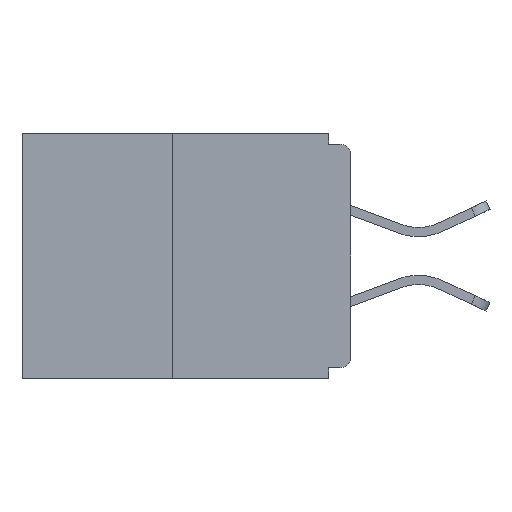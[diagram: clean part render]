
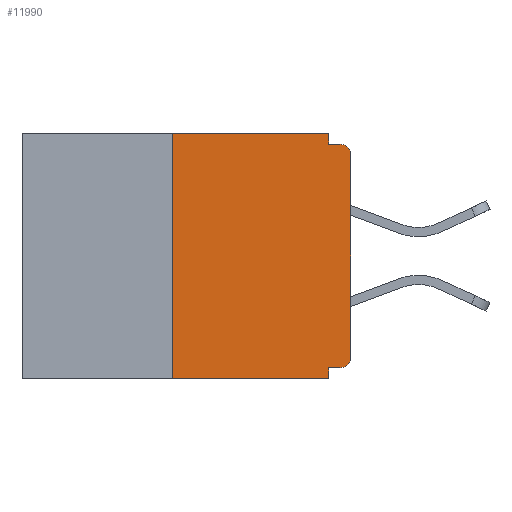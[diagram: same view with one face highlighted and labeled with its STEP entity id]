
A CAD part, left-side view. The second image highlights one B-rep face of the part: STEP entity #11990.
In plain terms, the highlighted planar face has unit normal (-1, 0, 0).
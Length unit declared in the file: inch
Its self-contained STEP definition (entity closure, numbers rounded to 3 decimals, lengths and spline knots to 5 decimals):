
#153 = ORIENTED_EDGE ( 'NONE', *, *, #921, .F. ) ;
#173 = CIRCLE ( 'NONE', #13445, 0.015 ) ;
#210 = LINE ( 'NONE', #9783, #8534 ) ;
#427 = EDGE_CURVE ( 'NONE', #8750, #3684, #10177, .T. ) ;
#473 = DIRECTION ( 'NONE',  ( 0., 0., -1. ) ) ;
#838 = FACE_OUTER_BOUND ( 'NONE', #8747, .T. ) ;
#877 = ORIENTED_EDGE ( 'NONE', *, *, #4428, .F. ) ;
#881 = ORIENTED_EDGE ( 'NONE', *, *, #7845, .T. ) ;
#921 = EDGE_CURVE ( 'NONE', #4093, #3684, #210, .T. ) ;
#939 = DIRECTION ( 'NONE',  ( 0., 0., -1. ) ) ;
#1078 = VECTOR ( 'NONE', #3060, 39.37008 ) ;
#1150 = DIRECTION ( 'NONE',  ( -1., 0., 0. ) ) ;
#1217 = EDGE_CURVE ( 'NONE', #6729, #9254, #11282, .T. ) ;
#1259 = VERTEX_POINT ( 'NONE', #10330 ) ;
#1319 = EDGE_CURVE ( 'NONE', #12414, #3350, #7712, .T. ) ;
#1530 = CARTESIAN_POINT ( 'NONE',  ( 0., 0., 0. ) ) ;
#1594 = DIRECTION ( 'NONE',  ( 0., 0., 1. ) ) ;
#1760 = ORIENTED_EDGE ( 'NONE', *, *, #1319, .T. ) ;
#1875 = CARTESIAN_POINT ( 'NONE',  ( 0., 0.46, -0.343 ) ) ;
#2273 = CARTESIAN_POINT ( 'NONE',  ( 0., 0.25, -0.343 ) ) ;
#2365 = VECTOR ( 'NONE', #11163, 39.37008 ) ;
#2523 = CARTESIAN_POINT ( 'NONE',  ( 0., 0.031, -0.343 ) ) ;
#2610 = LINE ( 'NONE', #9800, #8626 ) ;
#2629 = VERTEX_POINT ( 'NONE', #4858 ) ;
#2998 = LINE ( 'NONE', #11138, #1078 ) ;
#3060 = DIRECTION ( 'NONE',  ( 0., 0., -1. ) ) ;
#3350 = VERTEX_POINT ( 'NONE', #5543 ) ;
#3530 = VERTEX_POINT ( 'NONE', #4426 ) ;
#3684 = VERTEX_POINT ( 'NONE', #2523 ) ;
#3957 = DIRECTION ( 'NONE',  ( 0., 0., -1. ) ) ;
#4093 = VERTEX_POINT ( 'NONE', #7667 ) ;
#4126 = ORIENTED_EDGE ( 'NONE', *, *, #11527, .F. ) ;
#4337 = LINE ( 'NONE', #5232, #5018 ) ;
#4426 = CARTESIAN_POINT ( 'NONE',  ( 0., 0.015, -0.328 ) ) ;
#4428 = EDGE_CURVE ( 'NONE', #3530, #4093, #4337, .T. ) ;
#4579 = EDGE_CURVE ( 'NONE', #2629, #6729, #2998, .T. ) ;
#4686 = CARTESIAN_POINT ( 'NONE',  ( 0., 0., -0.313 ) ) ;
#4858 = CARTESIAN_POINT ( 'NONE',  ( 0., 0.031, 0. ) ) ;
#5018 = VECTOR ( 'NONE', #8340, 39.37008 ) ;
#5019 = DIRECTION ( 'NONE',  ( 0., -1., 0. ) ) ;
#5079 = ORIENTED_EDGE ( 'NONE', *, *, #4579, .F. ) ;
#5232 = CARTESIAN_POINT ( 'NONE',  ( 0., 0., -0.328 ) ) ;
#5283 = CARTESIAN_POINT ( 'NONE',  ( 0., 0.015, -0.313 ) ) ;
#5287 = ORIENTED_EDGE ( 'NONE', *, *, #1217, .F. ) ;
#5297 = DIRECTION ( 'NONE',  ( 0., 0., -1. ) ) ;
#5543 = CARTESIAN_POINT ( 'NONE',  ( 0., 0., -0.03 ) ) ;
#5709 = VECTOR ( 'NONE', #5019, 39.37008 ) ;
#5776 = CARTESIAN_POINT ( 'NONE',  ( 0., 0.031, -0.015 ) ) ;
#5864 = CARTESIAN_POINT ( 'NONE',  ( 0., 0.46, 0. ) ) ;
#6062 = CARTESIAN_POINT ( 'NONE',  ( 0., 0., -0.015 ) ) ;
#6729 = VERTEX_POINT ( 'NONE', #5776 ) ;
#6883 = PLANE ( 'NONE',  #8600 ) ;
#7035 = VECTOR ( 'NONE', #13404, 39.37008 ) ;
#7193 = DIRECTION ( 'NONE',  ( -1., 0., 0. ) ) ;
#7339 = CARTESIAN_POINT ( 'NONE',  ( 0., 0.015, -0.03 ) ) ;
#7372 = CARTESIAN_POINT ( 'NONE',  ( 0., 0.015, -0.015 ) ) ;
#7457 = VECTOR ( 'NONE', #1594, 39.37008 ) ;
#7548 = ORIENTED_EDGE ( 'NONE', *, *, #427, .T. ) ;
#7667 = CARTESIAN_POINT ( 'NONE',  ( 0., 0.031, -0.328 ) ) ;
#7712 = LINE ( 'NONE', #1530, #7457 ) ;
#7845 = EDGE_CURVE ( 'NONE', #3350, #9254, #12036, .T. ) ;
#8340 = DIRECTION ( 'NONE',  ( 0., 1., 0. ) ) ;
#8394 = ORIENTED_EDGE ( 'NONE', *, *, #10616, .T. ) ;
#8534 = VECTOR ( 'NONE', #473, 39.37008 ) ;
#8600 = AXIS2_PLACEMENT_3D ( 'NONE', #5864, #10004, #3957 ) ;
#8626 = VECTOR ( 'NONE', #11905, 39.37008 ) ;
#8747 = EDGE_LOOP ( 'NONE', ( #4126, #9163, #7548, #153, #877, #8394, #1760, #881, #5287, #5079 ) ) ;
#8750 = VERTEX_POINT ( 'NONE', #2273 ) ;
#9163 = ORIENTED_EDGE ( 'NONE', *, *, #13054, .F. ) ;
#9201 = LINE ( 'NONE', #11239, #2365 ) ;
#9254 = VERTEX_POINT ( 'NONE', #7372 ) ;
#9783 = CARTESIAN_POINT ( 'NONE',  ( 0., 0.031, -0.343 ) ) ;
#9800 = CARTESIAN_POINT ( 'NONE',  ( 0., 0.25, 0. ) ) ;
#10004 = DIRECTION ( 'NONE',  ( 1., 0., 0. ) ) ;
#10177 = LINE ( 'NONE', #1875, #5709 ) ;
#10330 = CARTESIAN_POINT ( 'NONE',  ( 0., 0.25, 0. ) ) ;
#10616 = EDGE_CURVE ( 'NONE', #3530, #12414, #173, .T. ) ;
#10952 = AXIS2_PLACEMENT_3D ( 'NONE', #7339, #1150, #5297 ) ;
#11138 = CARTESIAN_POINT ( 'NONE',  ( 0., 0.031, 0. ) ) ;
#11163 = DIRECTION ( 'NONE',  ( 0., -1., 0. ) ) ;
#11239 = CARTESIAN_POINT ( 'NONE',  ( 0., 0.46, 0. ) ) ;
#11282 = LINE ( 'NONE', #6062, #7035 ) ;
#11527 = EDGE_CURVE ( 'NONE', #1259, #2629, #9201, .T. ) ;
#11905 = DIRECTION ( 'NONE',  ( 0., 0., 1. ) ) ;
#11990 = ADVANCED_FACE ( 'NONE', ( #838 ), #6883, .F. ) ;
#12036 = CIRCLE ( 'NONE', #10952, 0.015 ) ;
#12414 = VERTEX_POINT ( 'NONE', #4686 ) ;
#13054 = EDGE_CURVE ( 'NONE', #8750, #1259, #2610, .T. ) ;
#13404 = DIRECTION ( 'NONE',  ( 0., -1., 0. ) ) ;
#13445 = AXIS2_PLACEMENT_3D ( 'NONE', #5283, #7193, #939 ) ;
